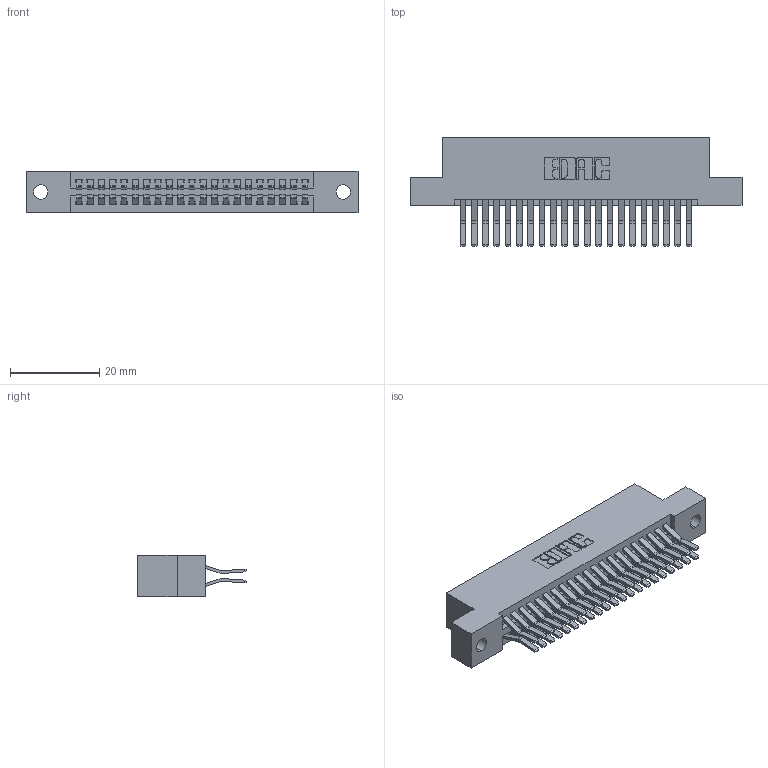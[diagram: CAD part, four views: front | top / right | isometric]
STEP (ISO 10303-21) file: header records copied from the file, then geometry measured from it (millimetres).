
FILE_DESCRIPTION (( 'STEP AP203' ), '1' );
FILE_NAME ('395-042-560-202.STEP', '2019-10-18T13:39:08', ( '' ), ( '' ), 'SwSTEP 2.0', 'SolidWorks 2016', '' );
FILE_SCHEMA (( 'CONFIG_CONTROL_DESIGN' ));
Length unit declared in the file: inch
Products named in the file (3): 345 Part_Flush Mounting Lugs - 0.128 Dia; 345-292-001_560 Tail; 395-042-560-202
Assembly tree (43 placements, depth 2):
  395-042-560-202
    345 Part_Flush Mounting Lugs - 0.128 Dia
    345-292-001_560 Tail  x42
Bounding box: 74.55 x 24.45 x 9.4 mm (x, y, z)
Volume: 7285.4 mm3; surface area: 10797.7 mm2
Topology: 43 solids, 43 shells, 2310 faces, 6851 edges, 4510 vertices
Faces by surface type: plane 1466, cylinder 844
Entity records: 19395 total; most frequent: CARTESIAN_POINT 3272, ORIENTED_EDGE 3206, DIRECTION 2915, EDGE_CURVE 1603, VECTOR 1383, LINE 1383, VERTEX_POINT 1066, AXIS2_PLACEMENT_3D 766
